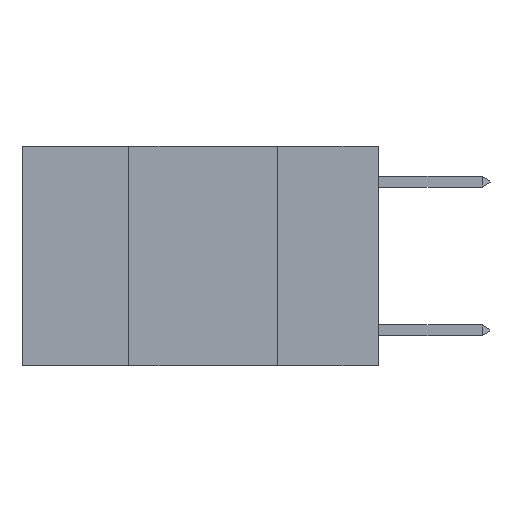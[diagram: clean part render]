
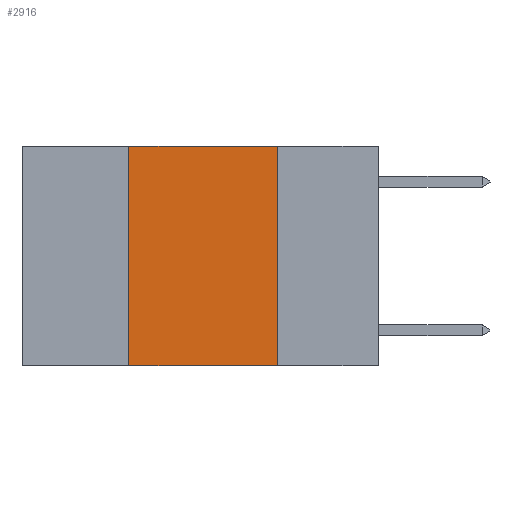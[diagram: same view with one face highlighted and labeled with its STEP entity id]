
A CAD part, left-side view. The second image highlights one B-rep face of the part: STEP entity #2916.
In plain terms, the highlighted planar face has unit normal (-1, 0, 0).
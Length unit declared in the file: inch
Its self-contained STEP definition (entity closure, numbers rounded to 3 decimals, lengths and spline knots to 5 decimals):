
#1404 = LINE ( 'NONE', #3336, #10780 ) ;
#2152 = EDGE_CURVE ( 'NONE', #8190, #10944, #6884, .T. ) ;
#2294 = CARTESIAN_POINT ( 'NONE',  ( 0., 0.42, 0. ) ) ;
#2748 = FACE_OUTER_BOUND ( 'NONE', #4979, .T. ) ;
#2769 = VECTOR ( 'NONE', #8640, 39.37008 ) ;
#2916 = ADVANCED_FACE ( 'NONE', ( #2748 ), #5017, .F. ) ;
#3307 = DIRECTION ( 'NONE',  ( 0., -1., 0. ) ) ;
#3336 = CARTESIAN_POINT ( 'NONE',  ( 0., 0.6, -0.37 ) ) ;
#3556 = DIRECTION ( 'NONE',  ( 0., -1., 0. ) ) ;
#4101 = LINE ( 'NONE', #4488, #8624 ) ;
#4177 = CARTESIAN_POINT ( 'NONE',  ( 0., 0.17, 0. ) ) ;
#4394 = VERTEX_POINT ( 'NONE', #9558 ) ;
#4488 = CARTESIAN_POINT ( 'NONE',  ( 0., 0.6, 0. ) ) ;
#4910 = DIRECTION ( 'NONE',  ( 0., 0., -1. ) ) ;
#4930 = DIRECTION ( 'NONE',  ( 1., 0., 0. ) ) ;
#4943 = CARTESIAN_POINT ( 'NONE',  ( 0., 0.6, 0. ) ) ;
#4979 = EDGE_LOOP ( 'NONE', ( #6696, #6964, #7128, #7167 ) ) ;
#5017 = PLANE ( 'NONE',  #8162 ) ;
#5101 = EDGE_CURVE ( 'NONE', #11093, #10944, #1404, .T. ) ;
#6303 = VECTOR ( 'NONE', #10814, 39.37008 ) ;
#6498 = EDGE_CURVE ( 'NONE', #4394, #8190, #4101, .T. ) ;
#6696 = ORIENTED_EDGE ( 'NONE', *, *, #2152, .F. ) ;
#6884 = LINE ( 'NONE', #10896, #6303 ) ;
#6964 = ORIENTED_EDGE ( 'NONE', *, *, #6498, .F. ) ;
#7128 = ORIENTED_EDGE ( 'NONE', *, *, #10291, .F. ) ;
#7167 = ORIENTED_EDGE ( 'NONE', *, *, #5101, .T. ) ;
#7980 = CARTESIAN_POINT ( 'NONE',  ( 0., 0.42, -0.37 ) ) ;
#8162 = AXIS2_PLACEMENT_3D ( 'NONE', #4943, #4930, #4910 ) ;
#8190 = VERTEX_POINT ( 'NONE', #4177 ) ;
#8594 = CARTESIAN_POINT ( 'NONE',  ( 0., 0.17, -0.37 ) ) ;
#8624 = VECTOR ( 'NONE', #3556, 39.37008 ) ;
#8640 = DIRECTION ( 'NONE',  ( 0., 0., 1. ) ) ;
#9558 = CARTESIAN_POINT ( 'NONE',  ( 0., 0.42, 0. ) ) ;
#9733 = LINE ( 'NONE', #2294, #2769 ) ;
#10291 = EDGE_CURVE ( 'NONE', #11093, #4394, #9733, .T. ) ;
#10780 = VECTOR ( 'NONE', #3307, 39.37008 ) ;
#10814 = DIRECTION ( 'NONE',  ( 0., 0., -1. ) ) ;
#10896 = CARTESIAN_POINT ( 'NONE',  ( 0., 0.17, 0. ) ) ;
#10944 = VERTEX_POINT ( 'NONE', #8594 ) ;
#11093 = VERTEX_POINT ( 'NONE', #7980 ) ;
